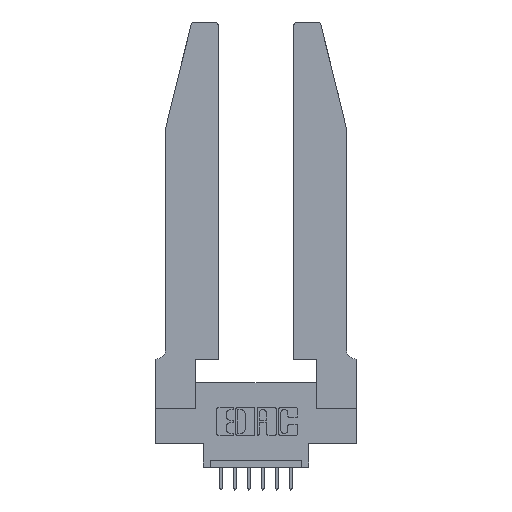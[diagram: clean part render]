
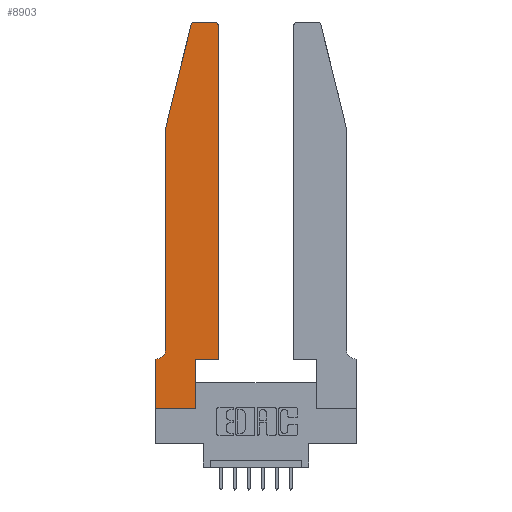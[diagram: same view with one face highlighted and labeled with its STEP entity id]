
A CAD part, top view. The second image highlights one B-rep face of the part: STEP entity #8903.
In plain terms, the highlighted planar face has unit normal (0, 0, 1).
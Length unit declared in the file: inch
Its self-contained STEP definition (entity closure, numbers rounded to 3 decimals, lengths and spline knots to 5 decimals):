
#16 = PLANE ( 'NONE',  #13340 ) ;
#130 = DIRECTION ( 'NONE',  ( -1., 0., 0. ) ) ;
#156 = EDGE_CURVE ( 'NONE', #7911, #7714, #11163, .T. ) ;
#306 = CARTESIAN_POINT ( 'NONE',  ( 0., 0.35, 0.37 ) ) ;
#364 = DIRECTION ( 'NONE',  ( 1., 0., 0. ) ) ;
#465 = VECTOR ( 'NONE', #13151, 39.37008 ) ;
#596 = VERTEX_POINT ( 'NONE', #306 ) ;
#789 = VECTOR ( 'NONE', #4956, 39.37008 ) ;
#822 = CARTESIAN_POINT ( 'NONE',  ( 0.25487, 2.72718, 0.37 ) ) ;
#1270 = CARTESIAN_POINT ( 'NONE',  ( 0.4505, 0.35, 0.37 ) ) ;
#1369 = DIRECTION ( 'NONE',  ( 0., -1., 0. ) ) ;
#1591 = EDGE_CURVE ( 'NONE', #6237, #14181, #6693, .T. ) ;
#1946 = AXIS2_PLACEMENT_3D ( 'NONE', #2383, #10163, #11279 ) ;
#2051 = AXIS2_PLACEMENT_3D ( 'NONE', #13602, #6986, #2386 ) ;
#2173 = CARTESIAN_POINT ( 'NONE',  ( 0.0055, 0.35, 0.37 ) ) ;
#2355 = EDGE_LOOP ( 'NONE', ( #8638, #10119, #3021, #3592, #11675, #11916, #9892, #13072, #6025, #5090, #9773, #10919 ) ) ;
#2361 = CARTESIAN_POINT ( 'NONE',  ( 0., 0.35, 0.37 ) ) ;
#2383 = CARTESIAN_POINT ( 'NONE',  ( 0.284, 2.72, 0.37 ) ) ;
#2386 = DIRECTION ( 'NONE',  ( -1., 0., 0. ) ) ;
#2418 = CARTESIAN_POINT ( 'NONE',  ( 0.0755, 0.42, 0.37 ) ) ;
#2570 = AXIS2_PLACEMENT_3D ( 'NONE', #11906, #4078, #8533 ) ;
#2637 = CARTESIAN_POINT ( 'NONE',  ( 0., 0., 0.37 ) ) ;
#2707 = VECTOR ( 'NONE', #364, 39.37008 ) ;
#2737 = VERTEX_POINT ( 'NONE', #5917 ) ;
#2840 = CARTESIAN_POINT ( 'NONE',  ( 0.4505, 0.35, 0.37 ) ) ;
#3021 = ORIENTED_EDGE ( 'NONE', *, *, #156, .T. ) ;
#3051 = CIRCLE ( 'NONE', #1946, 0.03 ) ;
#3568 = CARTESIAN_POINT ( 'NONE',  ( 0., 0., 0.37 ) ) ;
#3591 = CARTESIAN_POINT ( 'NONE',  ( 0., 0., 0.37 ) ) ;
#3592 = ORIENTED_EDGE ( 'NONE', *, *, #5440, .T. ) ;
#3720 = VECTOR ( 'NONE', #1369, 39.37008 ) ;
#3807 = VECTOR ( 'NONE', #13797, 39.37008 ) ;
#3819 = CARTESIAN_POINT ( 'NONE',  ( 0.0755, 2., 0.37 ) ) ;
#3843 = VERTEX_POINT ( 'NONE', #2418 ) ;
#3850 = EDGE_CURVE ( 'NONE', #10408, #10409, #11862, .T. ) ;
#4078 = DIRECTION ( 'NONE',  ( 0., 0., 1. ) ) ;
#4267 = CARTESIAN_POINT ( 'NONE',  ( 0.2865, 0.35, 0.37 ) ) ;
#4378 = CARTESIAN_POINT ( 'NONE',  ( 0.2865, 0., 0.37 ) ) ;
#4431 = CARTESIAN_POINT ( 'NONE',  ( 0.4205, 2.75, 0.37 ) ) ;
#4467 = EDGE_CURVE ( 'NONE', #6679, #6237, #13017, .T. ) ;
#4896 = LINE ( 'NONE', #11939, #9746 ) ;
#4956 = DIRECTION ( 'NONE',  ( -0.239, -0.971, 0. ) ) ;
#5090 = ORIENTED_EDGE ( 'NONE', *, *, #10032, .T. ) ;
#5166 = DIRECTION ( 'NONE',  ( 0., -1., 0. ) ) ;
#5440 = EDGE_CURVE ( 'NONE', #7714, #3843, #4896, .T. ) ;
#5917 = CARTESIAN_POINT ( 'NONE',  ( 0.4505, 2.72, 0.37 ) ) ;
#6025 = ORIENTED_EDGE ( 'NONE', *, *, #1591, .T. ) ;
#6218 = FACE_OUTER_BOUND ( 'NONE', #2355, .T. ) ;
#6237 = VERTEX_POINT ( 'NONE', #4378 ) ;
#6679 = VERTEX_POINT ( 'NONE', #3591 ) ;
#6693 = LINE ( 'NONE', #4267, #465 ) ;
#6773 = CARTESIAN_POINT ( 'NONE',  ( 0.2605, 2.75, 0.37 ) ) ;
#6986 = DIRECTION ( 'NONE',  ( 0., 0., -1. ) ) ;
#7714 = VERTEX_POINT ( 'NONE', #12488 ) ;
#7731 = EDGE_CURVE ( 'NONE', #3843, #13095, #9510, .T. ) ;
#7762 = DIRECTION ( 'NONE',  ( 0., 0., 1. ) ) ;
#7772 = LINE ( 'NONE', #2840, #13663 ) ;
#7800 = DIRECTION ( 'NONE',  ( 1., 0., 0. ) ) ;
#7911 = VERTEX_POINT ( 'NONE', #822 ) ;
#7950 = CARTESIAN_POINT ( 'NONE',  ( 0.4505, 0.35, 0.37 ) ) ;
#8533 = DIRECTION ( 'NONE',  ( 1., 0., 0. ) ) ;
#8544 = EDGE_CURVE ( 'NONE', #12206, #2737, #7772, .T. ) ;
#8638 = ORIENTED_EDGE ( 'NONE', *, *, #3850, .T. ) ;
#8889 = VECTOR ( 'NONE', #130, 39.37008 ) ;
#8903 = ADVANCED_FACE ( 'NONE', ( #6218 ), #16, .T. ) ;
#8914 = CARTESIAN_POINT ( 'NONE',  ( 0.0755, 0.35, 0.37 ) ) ;
#9032 = CARTESIAN_POINT ( 'NONE',  ( 0.2865, 0.35, 0.37 ) ) ;
#9303 = CIRCLE ( 'NONE', #2570, 0.03 ) ;
#9435 = VECTOR ( 'NONE', #13559, 39.37008 ) ;
#9510 = CIRCLE ( 'NONE', #2051, 0.07 ) ;
#9638 = LINE ( 'NONE', #3568, #3720 ) ;
#9746 = VECTOR ( 'NONE', #5166, 39.37008 ) ;
#9773 = ORIENTED_EDGE ( 'NONE', *, *, #8544, .T. ) ;
#9858 = EDGE_CURVE ( 'NONE', #2737, #10408, #9303, .T. ) ;
#9892 = ORIENTED_EDGE ( 'NONE', *, *, #12384, .T. ) ;
#10032 = EDGE_CURVE ( 'NONE', #14181, #12206, #11563, .T. ) ;
#10119 = ORIENTED_EDGE ( 'NONE', *, *, #11857, .T. ) ;
#10163 = DIRECTION ( 'NONE',  ( 0., 0., 1. ) ) ;
#10408 = VERTEX_POINT ( 'NONE', #4431 ) ;
#10409 = VERTEX_POINT ( 'NONE', #12197 ) ;
#10773 = DIRECTION ( 'NONE',  ( 0., 1., 0. ) ) ;
#10919 = ORIENTED_EDGE ( 'NONE', *, *, #9858, .T. ) ;
#11163 = LINE ( 'NONE', #3819, #789 ) ;
#11279 = DIRECTION ( 'NONE',  ( 1., 0., 0. ) ) ;
#11563 = LINE ( 'NONE', #7950, #2707 ) ;
#11675 = ORIENTED_EDGE ( 'NONE', *, *, #7731, .T. ) ;
#11699 = LINE ( 'NONE', #8914, #9435 ) ;
#11857 = EDGE_CURVE ( 'NONE', #10409, #7911, #3051, .T. ) ;
#11862 = LINE ( 'NONE', #6773, #8889 ) ;
#11906 = CARTESIAN_POINT ( 'NONE',  ( 0.4205, 2.72, 0.37 ) ) ;
#11916 = ORIENTED_EDGE ( 'NONE', *, *, #13508, .T. ) ;
#11939 = CARTESIAN_POINT ( 'NONE',  ( 0.0755, 2., 0.37 ) ) ;
#12197 = CARTESIAN_POINT ( 'NONE',  ( 0.284, 2.75, 0.37 ) ) ;
#12206 = VERTEX_POINT ( 'NONE', #1270 ) ;
#12384 = EDGE_CURVE ( 'NONE', #596, #6679, #9638, .T. ) ;
#12488 = CARTESIAN_POINT ( 'NONE',  ( 0.0755, 2., 0.37 ) ) ;
#13017 = LINE ( 'NONE', #2637, #3807 ) ;
#13072 = ORIENTED_EDGE ( 'NONE', *, *, #4467, .T. ) ;
#13095 = VERTEX_POINT ( 'NONE', #2173 ) ;
#13151 = DIRECTION ( 'NONE',  ( 0., 1., 0. ) ) ;
#13340 = AXIS2_PLACEMENT_3D ( 'NONE', #2361, #7762, #7800 ) ;
#13508 = EDGE_CURVE ( 'NONE', #13095, #596, #11699, .T. ) ;
#13559 = DIRECTION ( 'NONE',  ( -1., 0., 0. ) ) ;
#13602 = CARTESIAN_POINT ( 'NONE',  ( 0.0055, 0.42, 0.37 ) ) ;
#13663 = VECTOR ( 'NONE', #10773, 39.37008 ) ;
#13797 = DIRECTION ( 'NONE',  ( 1., 0., 0. ) ) ;
#14181 = VERTEX_POINT ( 'NONE', #9032 ) ;
